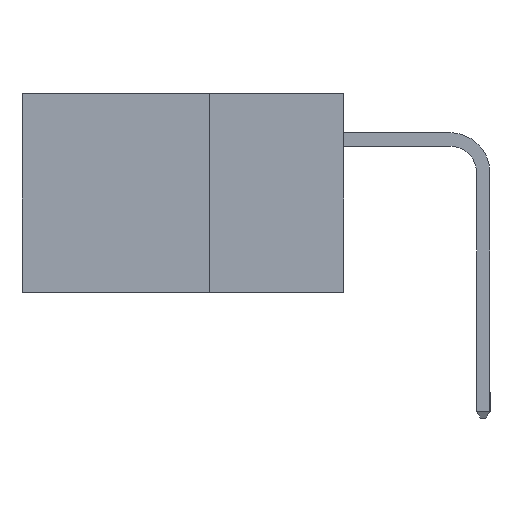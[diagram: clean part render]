
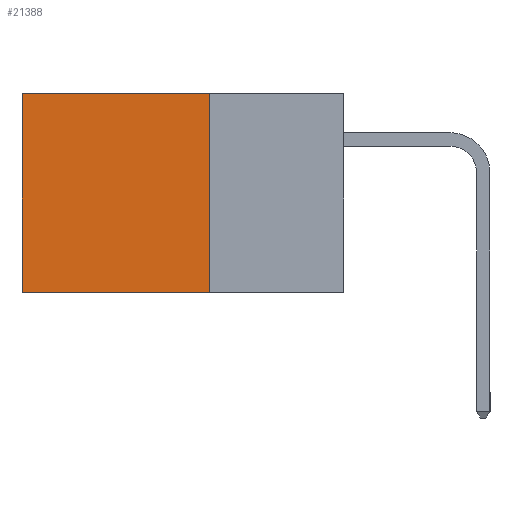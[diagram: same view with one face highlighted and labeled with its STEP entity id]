
A CAD part, left-side view. The second image highlights one B-rep face of the part: STEP entity #21388.
In plain terms, the highlighted planar face has unit normal (-1, 0, 0).
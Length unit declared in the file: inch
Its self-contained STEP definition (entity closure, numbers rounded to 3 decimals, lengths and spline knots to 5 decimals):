
#197 = EDGE_CURVE ( 'NONE', #15411, #3588, #16848, .T. ) ;
#222 = CARTESIAN_POINT ( 'NONE',  ( 0.298, 0.6, -0.37 ) ) ;
#1430 = DIRECTION ( 'NONE',  ( 0., 0., -1. ) ) ;
#1589 = ORIENTED_EDGE ( 'NONE', *, *, #14366, .F. ) ;
#2364 = DIRECTION ( 'NONE',  ( 1., 0., 0. ) ) ;
#3588 = VERTEX_POINT ( 'NONE', #222 ) ;
#4043 = CARTESIAN_POINT ( 'NONE',  ( 0.298, 0.25, 0. ) ) ;
#4578 = CARTESIAN_POINT ( 'NONE',  ( 0.298, 0.25, 0. ) ) ;
#5117 = LINE ( 'NONE', #4043, #13709 ) ;
#6074 = FACE_OUTER_BOUND ( 'NONE', #20874, .T. ) ;
#6866 = VERTEX_POINT ( 'NONE', #18680 ) ;
#7547 = CARTESIAN_POINT ( 'NONE',  ( 0.298, 0.6, 0. ) ) ;
#7823 = LINE ( 'NONE', #13352, #20852 ) ;
#8716 = ORIENTED_EDGE ( 'NONE', *, *, #197, .T. ) ;
#9643 = DIRECTION ( 'NONE',  ( 0., 0., -1. ) ) ;
#9901 = DIRECTION ( 'NONE',  ( 0., 1., 0. ) ) ;
#12597 = CARTESIAN_POINT ( 'NONE',  ( 0.298, 0.25, 0. ) ) ;
#12615 = VECTOR ( 'NONE', #9643, 39.37008 ) ;
#12677 = VERTEX_POINT ( 'NONE', #18060 ) ;
#13173 = CARTESIAN_POINT ( 'NONE',  ( 0.298, 0.6, 0. ) ) ;
#13352 = CARTESIAN_POINT ( 'NONE',  ( 0.298, 0.25, -0.37 ) ) ;
#13709 = VECTOR ( 'NONE', #15957, 39.37008 ) ;
#14332 = DIRECTION ( 'NONE',  ( 0., 0., -1. ) ) ;
#14366 = EDGE_CURVE ( 'NONE', #6866, #3588, #7823, .T. ) ;
#14430 = ORIENTED_EDGE ( 'NONE', *, *, #20743, .T. ) ;
#14930 = EDGE_CURVE ( 'NONE', #12677, #6866, #21593, .T. ) ;
#15411 = VERTEX_POINT ( 'NONE', #7547 ) ;
#15928 = ORIENTED_EDGE ( 'NONE', *, *, #14930, .F. ) ;
#15957 = DIRECTION ( 'NONE',  ( 0., 1., 0. ) ) ;
#16848 = LINE ( 'NONE', #13173, #17377 ) ;
#17377 = VECTOR ( 'NONE', #1430, 39.37008 ) ;
#17611 = PLANE ( 'NONE',  #19270 ) ;
#18060 = CARTESIAN_POINT ( 'NONE',  ( 0.298, 0.25, 0. ) ) ;
#18680 = CARTESIAN_POINT ( 'NONE',  ( 0.298, 0.25, -0.37 ) ) ;
#19270 = AXIS2_PLACEMENT_3D ( 'NONE', #12597, #2364, #14332 ) ;
#20743 = EDGE_CURVE ( 'NONE', #12677, #15411, #5117, .T. ) ;
#20852 = VECTOR ( 'NONE', #9901, 39.37008 ) ;
#20874 = EDGE_LOOP ( 'NONE', ( #8716, #1589, #15928, #14430 ) ) ;
#21388 = ADVANCED_FACE ( 'NONE', ( #6074 ), #17611, .F. ) ;
#21593 = LINE ( 'NONE', #4578, #12615 ) ;
